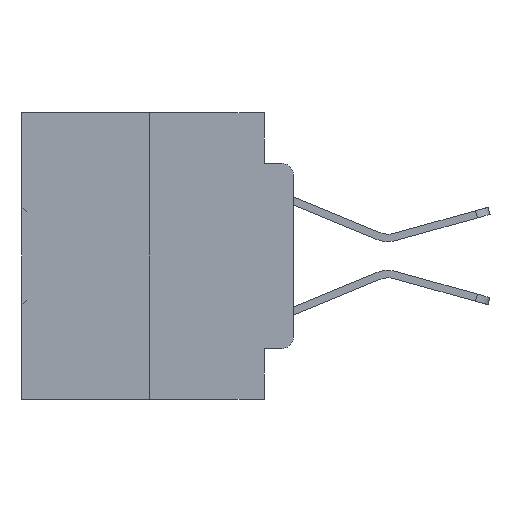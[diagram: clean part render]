
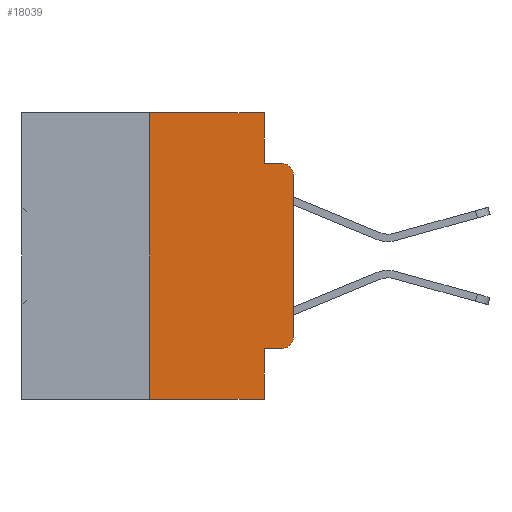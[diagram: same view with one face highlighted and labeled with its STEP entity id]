
A CAD part, left-side view. The second image highlights one B-rep face of the part: STEP entity #18039.
In plain terms, the highlighted planar face has unit normal (-1, 0, 0).
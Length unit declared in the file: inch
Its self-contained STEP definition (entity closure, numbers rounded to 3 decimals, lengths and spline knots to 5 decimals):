
#621 = ORIENTED_EDGE ( 'NONE', *, *, #14418, .F. ) ;
#996 = DIRECTION ( 'NONE',  ( 0., -1., 0. ) ) ;
#1796 = CARTESIAN_POINT ( 'NONE',  ( 0., 0., 0. ) ) ;
#1974 = LINE ( 'NONE', #34581, #24977 ) ;
#2419 = ORIENTED_EDGE ( 'NONE', *, *, #23939, .F. ) ;
#2437 = CARTESIAN_POINT ( 'NONE',  ( 0., 0., -0.3915 ) ) ;
#3364 = CARTESIAN_POINT ( 'NONE',  ( 0., 0.02, -0.1085 ) ) ;
#4056 = VECTOR ( 'NONE', #996, 39.37008 ) ;
#4151 = VERTEX_POINT ( 'NONE', #28373 ) ;
#4976 = LINE ( 'NONE', #28742, #6258 ) ;
#4981 = CARTESIAN_POINT ( 'NONE',  ( 0., 0.473, 0. ) ) ;
#5466 = VERTEX_POINT ( 'NONE', #2437 ) ;
#6258 = VECTOR ( 'NONE', #26917, 39.37008 ) ;
#6924 = ORIENTED_EDGE ( 'NONE', *, *, #16044, .F. ) ;
#7001 = VERTEX_POINT ( 'NONE', #28453 ) ;
#7013 = CARTESIAN_POINT ( 'NONE',  ( 0., 0.473, 0. ) ) ;
#7565 = CARTESIAN_POINT ( 'NONE',  ( 0., 0.02, -0.4115 ) ) ;
#7649 = CARTESIAN_POINT ( 'NONE',  ( 0., 0.02, -0.3915 ) ) ;
#8008 = DIRECTION ( 'NONE',  ( 0., 0., -1. ) ) ;
#8402 = CARTESIAN_POINT ( 'NONE',  ( 0., 0.051, 0. ) ) ;
#8648 = EDGE_CURVE ( 'NONE', #17862, #31339, #12074, .T. ) ;
#8982 = ORIENTED_EDGE ( 'NONE', *, *, #33742, .T. ) ;
#9543 = VECTOR ( 'NONE', #24378, 39.37008 ) ;
#10063 = EDGE_CURVE ( 'NONE', #22958, #30769, #31480, .T. ) ;
#10271 = EDGE_CURVE ( 'NONE', #7001, #4151, #1974, .T. ) ;
#10495 = ORIENTED_EDGE ( 'NONE', *, *, #10271, .F. ) ;
#10996 = DIRECTION ( 'NONE',  ( 0., 0., -1. ) ) ;
#11014 = VERTEX_POINT ( 'NONE', #26141 ) ;
#11708 = VECTOR ( 'NONE', #25324, 39.37008 ) ;
#12007 = CARTESIAN_POINT ( 'NONE',  ( 0., 0.25, -0.5 ) ) ;
#12074 = CIRCLE ( 'NONE', #32549, 0.02 ) ;
#12304 = DIRECTION ( 'NONE',  ( 0., 0., -1. ) ) ;
#12944 = CIRCLE ( 'NONE', #28524, 0.02 ) ;
#12984 = EDGE_CURVE ( 'NONE', #5466, #17862, #14828, .T. ) ;
#14335 = DIRECTION ( 'NONE',  ( 0., -1., 0. ) ) ;
#14418 = EDGE_CURVE ( 'NONE', #20138, #11014, #19055, .T. ) ;
#14575 = CARTESIAN_POINT ( 'NONE',  ( 0., 0.25, 0. ) ) ;
#14828 = LINE ( 'NONE', #1796, #21767 ) ;
#15531 = DIRECTION ( 'NONE',  ( 0., 0., 1. ) ) ;
#15724 = EDGE_LOOP ( 'NONE', ( #30539, #18150, #2419, #10495, #6924, #621, #8982, #20631, #26813, #20715 ) ) ;
#15895 = CARTESIAN_POINT ( 'NONE',  ( 0., 0., -0.1085 ) ) ;
#16044 = EDGE_CURVE ( 'NONE', #11014, #7001, #22517, .T. ) ;
#16440 = VECTOR ( 'NONE', #10996, 39.37008 ) ;
#16834 = AXIS2_PLACEMENT_3D ( 'NONE', #7013, #17804, #20713 ) ;
#17804 = DIRECTION ( 'NONE',  ( 1., 0., 0. ) ) ;
#17862 = VERTEX_POINT ( 'NONE', #15895 ) ;
#18039 = ADVANCED_FACE ( 'NONE', ( #27128 ), #33549, .F. ) ;
#18150 = ORIENTED_EDGE ( 'NONE', *, *, #8648, .T. ) ;
#19055 = LINE ( 'NONE', #14575, #11708 ) ;
#19177 = DIRECTION ( 'NONE',  ( -1., 0., 0. ) ) ;
#19611 = VERTEX_POINT ( 'NONE', #29086 ) ;
#20138 = VERTEX_POINT ( 'NONE', #12007 ) ;
#20631 = ORIENTED_EDGE ( 'NONE', *, *, #26910, .F. ) ;
#20713 = DIRECTION ( 'NONE',  ( 0., 0., -1. ) ) ;
#20715 = ORIENTED_EDGE ( 'NONE', *, *, #33921, .T. ) ;
#21767 = VECTOR ( 'NONE', #15531, 39.37008 ) ;
#22517 = LINE ( 'NONE', #4981, #9543 ) ;
#22525 = DIRECTION ( 'NONE',  ( 0., 0., -1. ) ) ;
#22958 = VERTEX_POINT ( 'NONE', #24441 ) ;
#23939 = EDGE_CURVE ( 'NONE', #4151, #31339, #32269, .T. ) ;
#24378 = DIRECTION ( 'NONE',  ( 0., -1., 0. ) ) ;
#24441 = CARTESIAN_POINT ( 'NONE',  ( 0., 0.051, -0.4115 ) ) ;
#24682 = LINE ( 'NONE', #8402, #16440 ) ;
#24977 = VECTOR ( 'NONE', #12304, 39.37008 ) ;
#25220 = CARTESIAN_POINT ( 'NONE',  ( 0., 0.051, -0.4115 ) ) ;
#25324 = DIRECTION ( 'NONE',  ( 0., 0., 1. ) ) ;
#25833 = VECTOR ( 'NONE', #14335, 39.37008 ) ;
#25927 = CARTESIAN_POINT ( 'NONE',  ( 0., 0.051, -0.0885 ) ) ;
#26141 = CARTESIAN_POINT ( 'NONE',  ( 0., 0.25, 0. ) ) ;
#26813 = ORIENTED_EDGE ( 'NONE', *, *, #10063, .T. ) ;
#26910 = EDGE_CURVE ( 'NONE', #22958, #19611, #24682, .T. ) ;
#26917 = DIRECTION ( 'NONE',  ( 0., -1., 0. ) ) ;
#27128 = FACE_OUTER_BOUND ( 'NONE', #15724, .T. ) ;
#27949 = DIRECTION ( 'NONE',  ( -1., 0., 0. ) ) ;
#28373 = CARTESIAN_POINT ( 'NONE',  ( 0., 0.051, -0.0885 ) ) ;
#28453 = CARTESIAN_POINT ( 'NONE',  ( 0., 0.051, 0. ) ) ;
#28524 = AXIS2_PLACEMENT_3D ( 'NONE', #7649, #19177, #8008 ) ;
#28742 = CARTESIAN_POINT ( 'NONE',  ( 0., 0.473, -0.5 ) ) ;
#29086 = CARTESIAN_POINT ( 'NONE',  ( 0., 0.051, -0.5 ) ) ;
#30539 = ORIENTED_EDGE ( 'NONE', *, *, #12984, .T. ) ;
#30769 = VERTEX_POINT ( 'NONE', #7565 ) ;
#31339 = VERTEX_POINT ( 'NONE', #31723 ) ;
#31480 = LINE ( 'NONE', #25220, #25833 ) ;
#31723 = CARTESIAN_POINT ( 'NONE',  ( 0., 0.02, -0.0885 ) ) ;
#32269 = LINE ( 'NONE', #25927, #4056 ) ;
#32549 = AXIS2_PLACEMENT_3D ( 'NONE', #3364, #27949, #22525 ) ;
#33549 = PLANE ( 'NONE',  #16834 ) ;
#33742 = EDGE_CURVE ( 'NONE', #20138, #19611, #4976, .T. ) ;
#33921 = EDGE_CURVE ( 'NONE', #30769, #5466, #12944, .T. ) ;
#34581 = CARTESIAN_POINT ( 'NONE',  ( 0., 0.051, 0. ) ) ;
